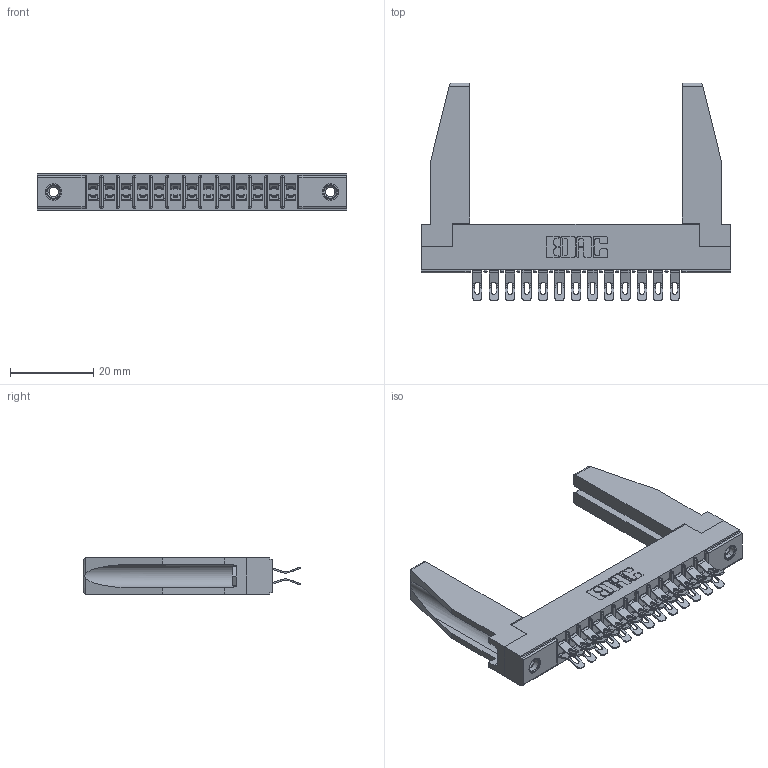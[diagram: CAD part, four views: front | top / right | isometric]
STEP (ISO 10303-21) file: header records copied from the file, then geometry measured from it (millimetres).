
FILE_DESCRIPTION (( 'STEP AP203' ), '1' );
FILE_NAME ('315-026-555-278.STEP', '2019-09-10T14:59:10', ( '' ), ( '' ), 'SwSTEP 2.0', 'SolidWorks 2016', '' );
FILE_SCHEMA (( 'CONFIG_CONTROL_DESIGN' ));
Length unit declared in the file: inch
Products named in the file (5): 315-026-555-278; 307-220-078; 305 Part_.156 Dia; 345-250-001_345-250-001-102; 305-290-001_555
Assembly tree (31 placements, depth 2):
  315-026-555-278
    305 Part_.156 Dia
    305-290-001_555  x26
    345-250-001_345-250-001-102  x2
    307-220-078  x2
Bounding box: 74.52 x 52.45 x 8.71 mm (x, y, z)
Volume: 8761.7 mm3; surface area: 12729.3 mm2
Topology: 31 solids, 31 shells, 1962 faces, 5781 edges, 3774 vertices
Faces by surface type: plane 984, cylinder 910, sphere 52, cone 12, torus 4
Entity records: 20669 total; most frequent: CARTESIAN_POINT 3445, ORIENTED_EDGE 3364, DIRECTION 3308, EDGE_CURVE 1682, LINE 1306, VECTOR 1306, VERTEX_POINT 1080, AXIS2_PLACEMENT_3D 1001
